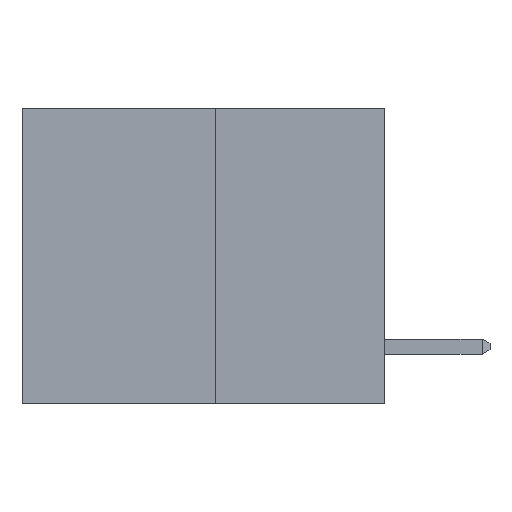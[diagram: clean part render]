
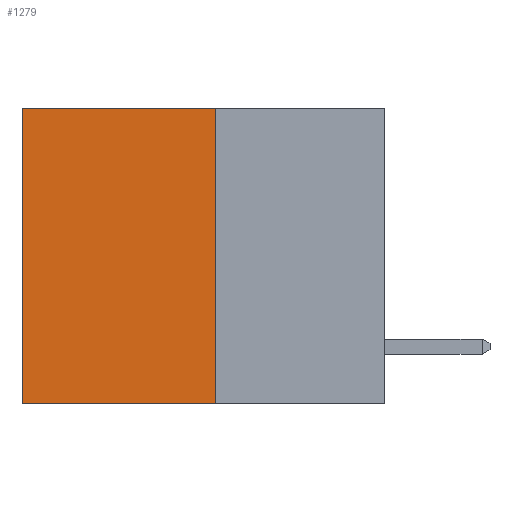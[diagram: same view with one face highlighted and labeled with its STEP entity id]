
A CAD part, left-side view. The second image highlights one B-rep face of the part: STEP entity #1279.
In plain terms, the highlighted planar face has unit normal (-1, 0, 0).
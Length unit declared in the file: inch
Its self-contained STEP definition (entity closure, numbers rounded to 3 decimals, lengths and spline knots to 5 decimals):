
#80 = FACE_OUTER_BOUND ( 'NONE', #6696, .T. ) ;
#576 = EDGE_CURVE ( 'NONE', #2313, #1288, #5817, .T. ) ;
#1066 = CARTESIAN_POINT ( 'NONE',  ( 0.3165, 0.28, 0. ) ) ;
#1279 = ADVANCED_FACE ( 'NONE', ( #80 ), #1887, .F. ) ;
#1288 = VERTEX_POINT ( 'NONE', #7397 ) ;
#1362 = DIRECTION ( 'NONE',  ( 0., 0., -1. ) ) ;
#1847 = VERTEX_POINT ( 'NONE', #6913 ) ;
#1887 = PLANE ( 'NONE',  #7509 ) ;
#2224 = EDGE_CURVE ( 'NONE', #1288, #4667, #5770, .T. ) ;
#2313 = VERTEX_POINT ( 'NONE', #7176 ) ;
#2597 = VECTOR ( 'NONE', #6433, 39.37008 ) ;
#2723 = CARTESIAN_POINT ( 'NONE',  ( 0.3165, 0.6, -0.49 ) ) ;
#3164 = CARTESIAN_POINT ( 'NONE',  ( 0.3165, 0.28, -0.49 ) ) ;
#3210 = LINE ( 'NONE', #3164, #7877 ) ;
#3698 = DIRECTION ( 'NONE',  ( 0., 1., 0. ) ) ;
#4071 = CARTESIAN_POINT ( 'NONE',  ( 0.3165, 0.28, -0.49 ) ) ;
#4161 = ORIENTED_EDGE ( 'NONE', *, *, #2224, .T. ) ;
#4386 = EDGE_CURVE ( 'NONE', #2313, #1847, #7364, .T. ) ;
#4577 = ORIENTED_EDGE ( 'NONE', *, *, #5829, .F. ) ;
#4667 = VERTEX_POINT ( 'NONE', #4981 ) ;
#4981 = CARTESIAN_POINT ( 'NONE',  ( 0.3165, 0.6, -0.49 ) ) ;
#5070 = VECTOR ( 'NONE', #6475, 39.37008 ) ;
#5770 = LINE ( 'NONE', #2723, #7202 ) ;
#5817 = LINE ( 'NONE', #1066, #5070 ) ;
#5829 = EDGE_CURVE ( 'NONE', #1847, #4667, #3210, .T. ) ;
#6392 = ORIENTED_EDGE ( 'NONE', *, *, #4386, .F. ) ;
#6433 = DIRECTION ( 'NONE',  ( 0., 0., -1. ) ) ;
#6475 = DIRECTION ( 'NONE',  ( 0., 1., 0. ) ) ;
#6696 = EDGE_LOOP ( 'NONE', ( #4161, #4577, #6392, #7666 ) ) ;
#6913 = CARTESIAN_POINT ( 'NONE',  ( 0.3165, 0.28, -0.49 ) ) ;
#6998 = DIRECTION ( 'NONE',  ( 0., 0., -1. ) ) ;
#7176 = CARTESIAN_POINT ( 'NONE',  ( 0.3165, 0.28, 0. ) ) ;
#7202 = VECTOR ( 'NONE', #6998, 39.37008 ) ;
#7352 = CARTESIAN_POINT ( 'NONE',  ( 0.3165, 0.28, -0.49 ) ) ;
#7364 = LINE ( 'NONE', #4071, #2597 ) ;
#7397 = CARTESIAN_POINT ( 'NONE',  ( 0.3165, 0.6, 0. ) ) ;
#7433 = DIRECTION ( 'NONE',  ( 1., 0., 0. ) ) ;
#7509 = AXIS2_PLACEMENT_3D ( 'NONE', #7352, #7433, #1362 ) ;
#7666 = ORIENTED_EDGE ( 'NONE', *, *, #576, .T. ) ;
#7877 = VECTOR ( 'NONE', #3698, 39.37008 ) ;
